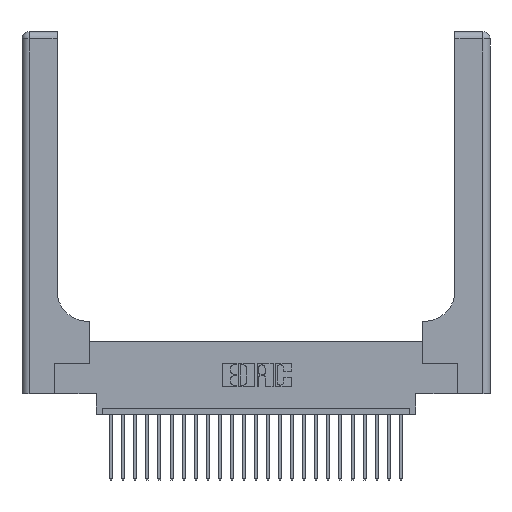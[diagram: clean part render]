
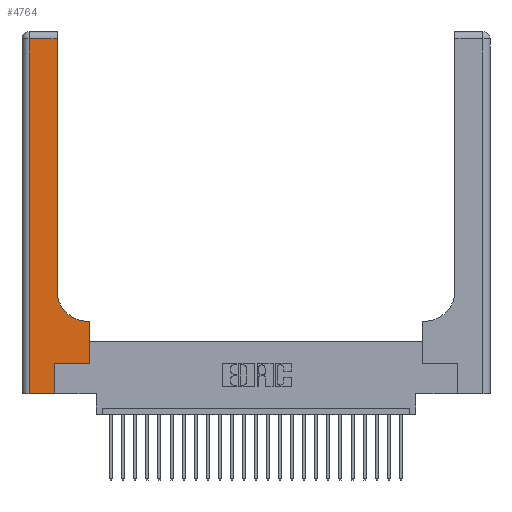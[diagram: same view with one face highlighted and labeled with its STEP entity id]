
A CAD part, top view. The second image highlights one B-rep face of the part: STEP entity #4764.
In plain terms, the highlighted planar face has unit normal (0, 0, 1).
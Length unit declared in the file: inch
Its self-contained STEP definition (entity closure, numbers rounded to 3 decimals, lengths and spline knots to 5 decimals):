
#477 = ORIENTED_EDGE ( 'NONE', *, *, #10795, .T. ) ;
#955 = CARTESIAN_POINT ( 'NONE',  ( 0.269, 0.25, 0.37 ) ) ;
#1013 = CARTESIAN_POINT ( 'NONE',  ( 0., 3., 0.37 ) ) ;
#1089 = VERTEX_POINT ( 'NONE', #1854 ) ;
#1128 = DIRECTION ( 'NONE',  ( 1., 0., 0. ) ) ;
#1847 = VERTEX_POINT ( 'NONE', #2055 ) ;
#1854 = CARTESIAN_POINT ( 'NONE',  ( 0.5585, 0.6, 0.37 ) ) ;
#1910 = CARTESIAN_POINT ( 'NONE',  ( 0., 0., 0.37 ) ) ;
#2055 = CARTESIAN_POINT ( 'NONE',  ( 0.06, 0., 0.37 ) ) ;
#2332 = VECTOR ( 'NONE', #1128, 39.37008 ) ;
#2649 = ORIENTED_EDGE ( 'NONE', *, *, #25139, .T. ) ;
#2979 = CARTESIAN_POINT ( 'NONE',  ( 0.5415, 0.6, 0.37 ) ) ;
#3299 = EDGE_CURVE ( 'NONE', #8725, #22701, #25234, .T. ) ;
#3443 = AXIS2_PLACEMENT_3D ( 'NONE', #1013, #21552, #9406 ) ;
#3504 = ORIENTED_EDGE ( 'NONE', *, *, #3299, .T. ) ;
#3900 = ORIENTED_EDGE ( 'NONE', *, *, #11062, .T. ) ;
#4005 = LINE ( 'NONE', #16252, #24385 ) ;
#4677 = CARTESIAN_POINT ( 'NONE',  ( 0.06, 2.94, 0.37 ) ) ;
#4764 = ADVANCED_FACE ( 'NONE', ( #14956 ), #7246, .F. ) ;
#4818 = EDGE_CURVE ( 'NONE', #15600, #15316, #12112, .T. ) ;
#5533 = VECTOR ( 'NONE', #13208, 39.37008 ) ;
#5841 = CARTESIAN_POINT ( 'NONE',  ( 0.269, 0., 0.37 ) ) ;
#6423 = CARTESIAN_POINT ( 'NONE',  ( 0.2915, 3., 0.37 ) ) ;
#6459 = DIRECTION ( 'NONE',  ( 0., 1., 0. ) ) ;
#6605 = DIRECTION ( 'NONE',  ( 0., 1., 0. ) ) ;
#6690 = CARTESIAN_POINT ( 'NONE',  ( 0., 2.94, 0.37 ) ) ;
#6715 = CARTESIAN_POINT ( 'NONE',  ( 0.5415, 0.85, 0.37 ) ) ;
#6925 = CARTESIAN_POINT ( 'NONE',  ( 0.269, 0.25, 0.37 ) ) ;
#7246 = PLANE ( 'NONE',  #3443 ) ;
#7353 = DIRECTION ( 'NONE',  ( 0., -1., 0. ) ) ;
#7428 = DIRECTION ( 'NONE',  ( -1., 0., 0. ) ) ;
#8725 = VERTEX_POINT ( 'NONE', #2979 ) ;
#9167 = EDGE_CURVE ( 'NONE', #20298, #1089, #4005, .T. ) ;
#9406 = DIRECTION ( 'NONE',  ( -1., 0., 0. ) ) ;
#9442 = LINE ( 'NONE', #1910, #22768 ) ;
#9789 = DIRECTION ( 'NONE',  ( -1., 0., 0. ) ) ;
#10795 = EDGE_CURVE ( 'NONE', #16085, #11909, #16981, .T. ) ;
#11062 = EDGE_CURVE ( 'NONE', #22701, #15600, #23028, .T. ) ;
#11163 = LINE ( 'NONE', #25444, #13995 ) ;
#11601 = VECTOR ( 'NONE', #6605, 39.37008 ) ;
#11909 = VERTEX_POINT ( 'NONE', #6925 ) ;
#12112 = LINE ( 'NONE', #6690, #19711 ) ;
#12349 = EDGE_CURVE ( 'NONE', #1089, #8725, #21056, .T. ) ;
#13208 = DIRECTION ( 'NONE',  ( 0., 1., 0. ) ) ;
#13587 = CARTESIAN_POINT ( 'NONE',  ( 0.2915, 0.6, 0.37 ) ) ;
#13995 = VECTOR ( 'NONE', #7353, 39.37008 ) ;
#14519 = EDGE_LOOP ( 'NONE', ( #3900, #18261, #2649, #19903, #477, #24281, #18464, #21739, #3504 ) ) ;
#14532 = CARTESIAN_POINT ( 'NONE',  ( 0.2915, 0.85, 0.37 ) ) ;
#14956 = FACE_OUTER_BOUND ( 'NONE', #14519, .T. ) ;
#15316 = VERTEX_POINT ( 'NONE', #4677 ) ;
#15550 = AXIS2_PLACEMENT_3D ( 'NONE', #6715, #16915, #23245 ) ;
#15600 = VERTEX_POINT ( 'NONE', #26079 ) ;
#16085 = VERTEX_POINT ( 'NONE', #5841 ) ;
#16252 = CARTESIAN_POINT ( 'NONE',  ( 0.5585, 0.25, 0.37 ) ) ;
#16399 = EDGE_CURVE ( 'NONE', #1847, #16085, #9442, .T. ) ;
#16915 = DIRECTION ( 'NONE',  ( 0., 0., -1. ) ) ;
#16981 = LINE ( 'NONE', #17277, #5533 ) ;
#17277 = CARTESIAN_POINT ( 'NONE',  ( 0.269, 0., 0.37 ) ) ;
#18261 = ORIENTED_EDGE ( 'NONE', *, *, #4818, .T. ) ;
#18307 = DIRECTION ( 'NONE',  ( 1., 0., 0. ) ) ;
#18464 = ORIENTED_EDGE ( 'NONE', *, *, #9167, .T. ) ;
#18493 = EDGE_CURVE ( 'NONE', #11909, #20298, #19894, .T. ) ;
#19711 = VECTOR ( 'NONE', #7428, 39.37008 ) ;
#19894 = LINE ( 'NONE', #955, #2332 ) ;
#19903 = ORIENTED_EDGE ( 'NONE', *, *, #16399, .T. ) ;
#20298 = VERTEX_POINT ( 'NONE', #24522 ) ;
#21056 = LINE ( 'NONE', #13587, #23907 ) ;
#21552 = DIRECTION ( 'NONE',  ( 0., 0., -1. ) ) ;
#21739 = ORIENTED_EDGE ( 'NONE', *, *, #12349, .T. ) ;
#22701 = VERTEX_POINT ( 'NONE', #14532 ) ;
#22768 = VECTOR ( 'NONE', #18307, 39.37008 ) ;
#23028 = LINE ( 'NONE', #6423, #11601 ) ;
#23245 = DIRECTION ( 'NONE',  ( 1., 0., 0. ) ) ;
#23907 = VECTOR ( 'NONE', #9789, 39.37008 ) ;
#24281 = ORIENTED_EDGE ( 'NONE', *, *, #18493, .T. ) ;
#24385 = VECTOR ( 'NONE', #6459, 39.37008 ) ;
#24522 = CARTESIAN_POINT ( 'NONE',  ( 0.5585, 0.25, 0.37 ) ) ;
#25139 = EDGE_CURVE ( 'NONE', #15316, #1847, #11163, .T. ) ;
#25234 = CIRCLE ( 'NONE', #15550, 0.25 ) ;
#25444 = CARTESIAN_POINT ( 'NONE',  ( 0.06, 3., 0.37 ) ) ;
#26079 = CARTESIAN_POINT ( 'NONE',  ( 0.2915, 2.94, 0.37 ) ) ;
